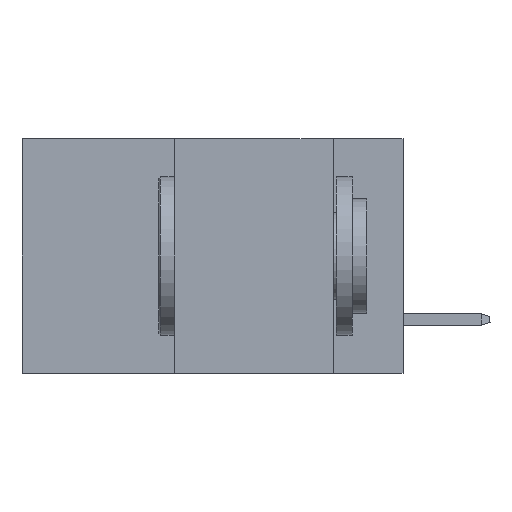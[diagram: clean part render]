
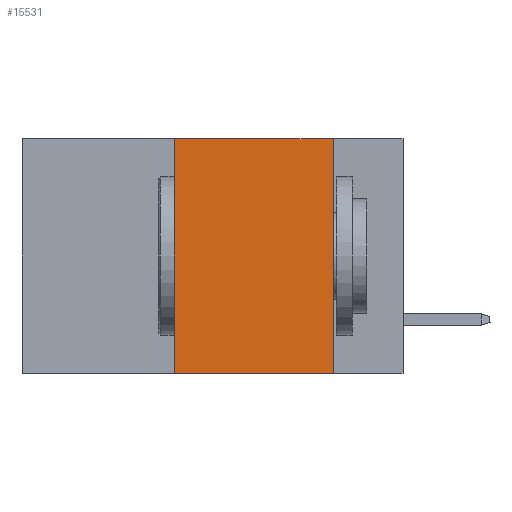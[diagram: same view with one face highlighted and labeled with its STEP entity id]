
A CAD part, left-side view. The second image highlights one B-rep face of the part: STEP entity #15531.
In plain terms, the highlighted planar face has unit normal (-1, 0, 0).
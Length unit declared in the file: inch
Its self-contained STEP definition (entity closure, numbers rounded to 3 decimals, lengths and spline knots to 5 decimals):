
#349 = VECTOR ( 'NONE', #5481, 39.37008 ) ;
#585 = CARTESIAN_POINT ( 'NONE',  ( 0., 0.36, -0.37 ) ) ;
#930 = VECTOR ( 'NONE', #2428, 39.37008 ) ;
#1473 = CARTESIAN_POINT ( 'NONE',  ( 0., 0.11, 0. ) ) ;
#2071 = VECTOR ( 'NONE', #14297, 39.37008 ) ;
#2407 = DIRECTION ( 'NONE',  ( 0., 0., -1. ) ) ;
#2428 = DIRECTION ( 'NONE',  ( 0., 0., -1. ) ) ;
#2639 = VERTEX_POINT ( 'NONE', #18663 ) ;
#2779 = FACE_OUTER_BOUND ( 'NONE', #10841, .T. ) ;
#2823 = CARTESIAN_POINT ( 'NONE',  ( 0., 0.11, -0.37 ) ) ;
#3066 = EDGE_CURVE ( 'NONE', #2639, #17291, #17078, .T. ) ;
#3830 = CARTESIAN_POINT ( 'NONE',  ( 0., 0.6, 0. ) ) ;
#4169 = PLANE ( 'NONE',  #9779 ) ;
#4426 = ORIENTED_EDGE ( 'NONE', *, *, #16304, .T. ) ;
#5481 = DIRECTION ( 'NONE',  ( 0., -1., 0. ) ) ;
#6284 = DIRECTION ( 'NONE',  ( 0., 0., 1. ) ) ;
#6763 = EDGE_CURVE ( 'NONE', #12017, #2639, #14984, .T. ) ;
#7125 = VERTEX_POINT ( 'NONE', #2823 ) ;
#7162 = LINE ( 'NONE', #11712, #349 ) ;
#8805 = DIRECTION ( 'NONE',  ( 1., 0., 0. ) ) ;
#9024 = ORIENTED_EDGE ( 'NONE', *, *, #6763, .F. ) ;
#9027 = VECTOR ( 'NONE', #6284, 39.37008 ) ;
#9779 = AXIS2_PLACEMENT_3D ( 'NONE', #10099, #8805, #2407 ) ;
#10099 = CARTESIAN_POINT ( 'NONE',  ( 0., 0.6, 0. ) ) ;
#10841 = EDGE_LOOP ( 'NONE', ( #14978, #16392, #9024, #4426 ) ) ;
#11712 = CARTESIAN_POINT ( 'NONE',  ( 0., 0.6, -0.37 ) ) ;
#12017 = VERTEX_POINT ( 'NONE', #585 ) ;
#12601 = EDGE_CURVE ( 'NONE', #17291, #7125, #17531, .T. ) ;
#12904 = CARTESIAN_POINT ( 'NONE',  ( 0., 0.11, 0. ) ) ;
#13417 = CARTESIAN_POINT ( 'NONE',  ( 0., 0.36, 0. ) ) ;
#14297 = DIRECTION ( 'NONE',  ( 0., -1., 0. ) ) ;
#14978 = ORIENTED_EDGE ( 'NONE', *, *, #12601, .F. ) ;
#14984 = LINE ( 'NONE', #13417, #9027 ) ;
#15531 = ADVANCED_FACE ( 'NONE', ( #2779 ), #4169, .F. ) ;
#16304 = EDGE_CURVE ( 'NONE', #12017, #7125, #7162, .T. ) ;
#16392 = ORIENTED_EDGE ( 'NONE', *, *, #3066, .F. ) ;
#17078 = LINE ( 'NONE', #3830, #2071 ) ;
#17291 = VERTEX_POINT ( 'NONE', #1473 ) ;
#17531 = LINE ( 'NONE', #12904, #930 ) ;
#18663 = CARTESIAN_POINT ( 'NONE',  ( 0., 0.36, 0. ) ) ;
